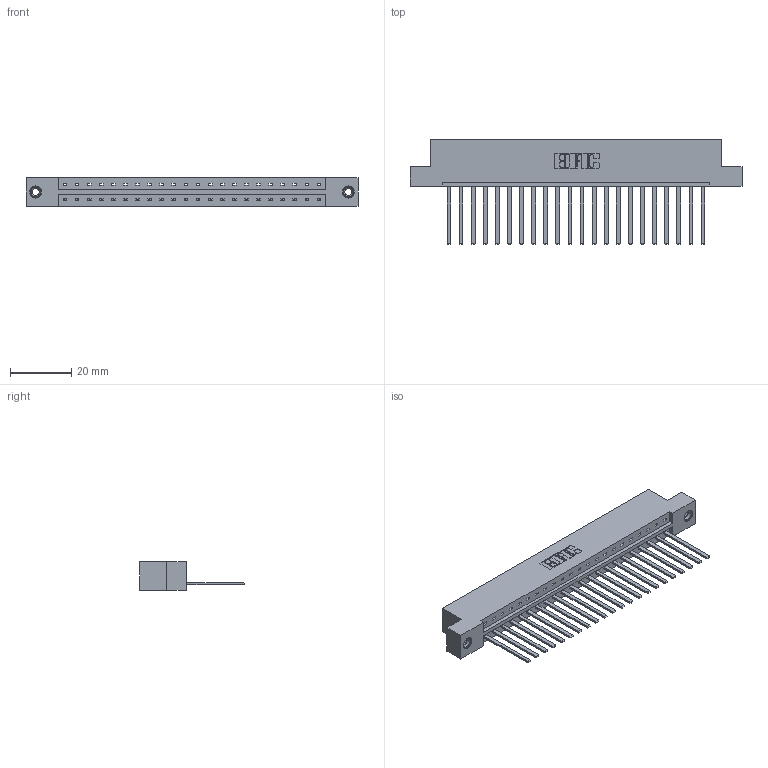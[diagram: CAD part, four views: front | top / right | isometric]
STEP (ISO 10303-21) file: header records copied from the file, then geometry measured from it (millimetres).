
FILE_DESCRIPTION (( 'STEP AP203' ), '1' );
FILE_NAME ('833-022-544-108.STEP', '2020-06-01T17:33:14', ( '' ), ( '' ), 'SwSTEP 2.0', 'SolidWorks 2020', '' );
FILE_SCHEMA (( 'CONFIG_CONTROL_DESIGN' ));
Length unit declared in the file: inch
Products named in the file (4): 345-292-001_345-293-144; 833-022-544-108; 345-250-001_345-250-003-102; 833 Part_Flush - .156 Dia - TI
Assembly tree (25 placements, depth 2):
  833-022-544-108
    833 Part_Flush - .156 Dia - TI
    345-292-001_345-293-144  x22
    345-250-001_345-250-003-102  x2
Bounding box: 108.71 x 34.3 x 9.4 mm (x, y, z)
Volume: 11015.8 mm3; surface area: 12642.3 mm2
Topology: 25 solids, 25 shells, 1318 faces, 3923 edges, 2578 vertices
Faces by surface type: plane 938, cylinder 364, cone 12, torus 4
Entity records: 17038 total; most frequent: CARTESIAN_POINT 2923, ORIENTED_EDGE 2874, DIRECTION 2535, EDGE_CURVE 1437, VECTOR 1293, LINE 1293, VERTEX_POINT 952, AXIS2_PLACEMENT_3D 621
